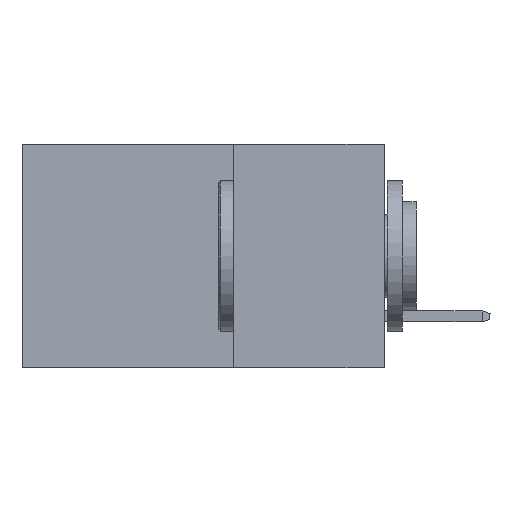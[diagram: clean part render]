
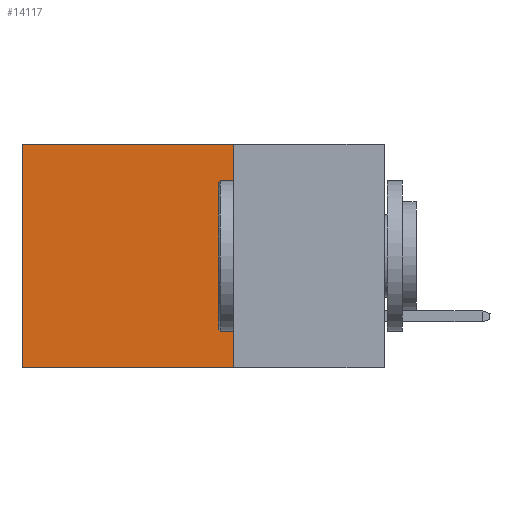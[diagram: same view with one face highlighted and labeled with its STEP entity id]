
A CAD part, left-side view. The second image highlights one B-rep face of the part: STEP entity #14117.
In plain terms, the highlighted planar face has unit normal (-1, 0, 0).
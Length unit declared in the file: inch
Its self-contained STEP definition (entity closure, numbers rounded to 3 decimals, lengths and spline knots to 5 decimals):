
#531 = CARTESIAN_POINT ( 'NONE',  ( 0.2615, 0.25, 0. ) ) ;
#647 = CARTESIAN_POINT ( 'NONE',  ( 0.2615, 0.25, -0.37 ) ) ;
#786 = LINE ( 'NONE', #531, #2854 ) ;
#890 = VERTEX_POINT ( 'NONE', #2874 ) ;
#1290 = ORIENTED_EDGE ( 'NONE', *, *, #10370, .T. ) ;
#1553 = VECTOR ( 'NONE', #3749, 39.37008 ) ;
#2357 = EDGE_LOOP ( 'NONE', ( #1290, #2679, #15904, #4958 ) ) ;
#2395 = LINE ( 'NONE', #7569, #1553 ) ;
#2679 = ORIENTED_EDGE ( 'NONE', *, *, #12146, .F. ) ;
#2694 = VERTEX_POINT ( 'NONE', #15687 ) ;
#2854 = VECTOR ( 'NONE', #16404, 39.37008 ) ;
#2874 = CARTESIAN_POINT ( 'NONE',  ( 0.2615, 0.6, 0. ) ) ;
#3050 = DIRECTION ( 'NONE',  ( 1., 0., 0. ) ) ;
#3189 = VECTOR ( 'NONE', #8464, 39.37008 ) ;
#3281 = CARTESIAN_POINT ( 'NONE',  ( 0.2615, 0.6, -0.37 ) ) ;
#3372 = CARTESIAN_POINT ( 'NONE',  ( 0.2615, 0.25, -0.37 ) ) ;
#3749 = DIRECTION ( 'NONE',  ( 0., 1., 0. ) ) ;
#4958 = ORIENTED_EDGE ( 'NONE', *, *, #5197, .T. ) ;
#5197 = EDGE_CURVE ( 'NONE', #2694, #890, #786, .T. ) ;
#5753 = VECTOR ( 'NONE', #8281, 39.37008 ) ;
#6362 = CARTESIAN_POINT ( 'NONE',  ( 0.2615, 0.6, -0.37 ) ) ;
#7501 = AXIS2_PLACEMENT_3D ( 'NONE', #13242, #3050, #12049 ) ;
#7569 = CARTESIAN_POINT ( 'NONE',  ( 0.2615, 0.25, -0.37 ) ) ;
#7881 = PLANE ( 'NONE',  #7501 ) ;
#8054 = FACE_OUTER_BOUND ( 'NONE', #2357, .T. ) ;
#8281 = DIRECTION ( 'NONE',  ( 0., 0., -1. ) ) ;
#8445 = LINE ( 'NONE', #647, #5753 ) ;
#8464 = DIRECTION ( 'NONE',  ( 0., 0., -1. ) ) ;
#10003 = VERTEX_POINT ( 'NONE', #6362 ) ;
#10370 = EDGE_CURVE ( 'NONE', #890, #10003, #16200, .T. ) ;
#12049 = DIRECTION ( 'NONE',  ( 0., 0., -1. ) ) ;
#12146 = EDGE_CURVE ( 'NONE', #12917, #10003, #2395, .T. ) ;
#12917 = VERTEX_POINT ( 'NONE', #3372 ) ;
#13242 = CARTESIAN_POINT ( 'NONE',  ( 0.2615, 0.25, -0.37 ) ) ;
#14117 = ADVANCED_FACE ( 'NONE', ( #8054 ), #7881, .F. ) ;
#14647 = EDGE_CURVE ( 'NONE', #2694, #12917, #8445, .T. ) ;
#15687 = CARTESIAN_POINT ( 'NONE',  ( 0.2615, 0.25, 0. ) ) ;
#15904 = ORIENTED_EDGE ( 'NONE', *, *, #14647, .F. ) ;
#16200 = LINE ( 'NONE', #3281, #3189 ) ;
#16404 = DIRECTION ( 'NONE',  ( 0., 1., 0. ) ) ;
